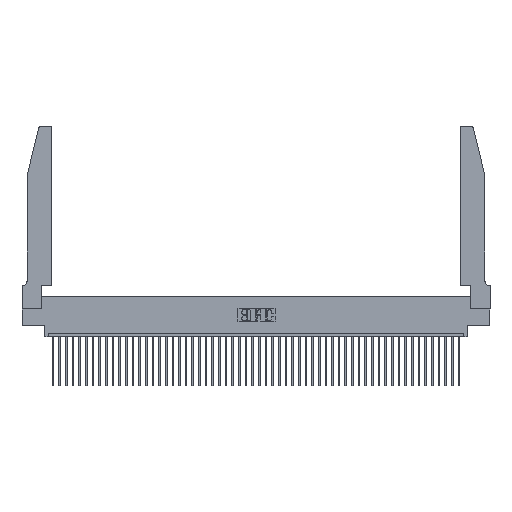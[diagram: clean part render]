
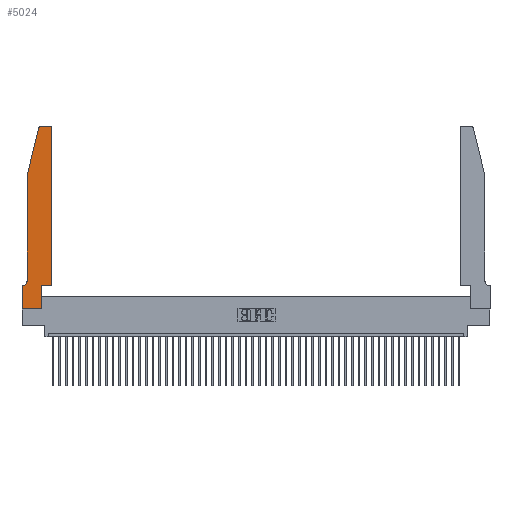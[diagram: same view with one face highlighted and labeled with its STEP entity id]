
A CAD part, top view. The second image highlights one B-rep face of the part: STEP entity #5024.
In plain terms, the highlighted planar face has unit normal (0, 0, 1).
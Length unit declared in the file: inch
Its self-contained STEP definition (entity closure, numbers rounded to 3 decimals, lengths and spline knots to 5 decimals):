
#981 = LINE ( 'NONE', #19259, #23423 ) ;
#1218 = CARTESIAN_POINT ( 'NONE',  ( 0.4205, 2.75, 0.37 ) ) ;
#2409 = LINE ( 'NONE', #38891, #30758 ) ;
#2956 = VERTEX_POINT ( 'NONE', #44778 ) ;
#4063 = LINE ( 'NONE', #10642, #10596 ) ;
#4858 = CARTESIAN_POINT ( 'NONE',  ( 0.0755, 0.42, 0.37 ) ) ;
#5024 = ADVANCED_FACE ( 'NONE', ( #37629 ), #31689, .T. ) ;
#5174 = AXIS2_PLACEMENT_3D ( 'NONE', #39821, #32008, #24219 ) ;
#5288 = CARTESIAN_POINT ( 'NONE',  ( 0.2605, 2.75, 0.37 ) ) ;
#5776 = ORIENTED_EDGE ( 'NONE', *, *, #29403, .T. ) ;
#6698 = CARTESIAN_POINT ( 'NONE',  ( 0.4505, 0.35, 0.37 ) ) ;
#6776 = EDGE_CURVE ( 'NONE', #11607, #11128, #981, .T. ) ;
#7155 = CARTESIAN_POINT ( 'NONE',  ( 0., 0., 0.37 ) ) ;
#7243 = EDGE_CURVE ( 'NONE', #45416, #43548, #16360, .T. ) ;
#7507 = VERTEX_POINT ( 'NONE', #24348 ) ;
#9375 = ORIENTED_EDGE ( 'NONE', *, *, #10533, .T. ) ;
#10142 = ORIENTED_EDGE ( 'NONE', *, *, #21286, .T. ) ;
#10409 = CARTESIAN_POINT ( 'NONE',  ( 0.25487, 2.72718, 0.37 ) ) ;
#10533 = EDGE_CURVE ( 'NONE', #43548, #13850, #2409, .T. ) ;
#10596 = VECTOR ( 'NONE', #25791, 39.37008 ) ;
#10642 = CARTESIAN_POINT ( 'NONE',  ( 0.2865, 0.35, 0.37 ) ) ;
#11128 = VERTEX_POINT ( 'NONE', #19359 ) ;
#11607 = VERTEX_POINT ( 'NONE', #10409 ) ;
#11941 = VECTOR ( 'NONE', #31706, 39.37008 ) ;
#12114 = ORIENTED_EDGE ( 'NONE', *, *, #33068, .T. ) ;
#12550 = LINE ( 'NONE', #29063, #44525 ) ;
#12596 = ORIENTED_EDGE ( 'NONE', *, *, #7243, .T. ) ;
#12612 = DIRECTION ( 'NONE',  ( 0., 0., 1. ) ) ;
#12664 = CIRCLE ( 'NONE', #46687, 0.03 ) ;
#13850 = VERTEX_POINT ( 'NONE', #18048 ) ;
#14382 = CARTESIAN_POINT ( 'NONE',  ( 0., 0.35, 0.37 ) ) ;
#15039 = ORIENTED_EDGE ( 'NONE', *, *, #22161, .T. ) ;
#15915 = DIRECTION ( 'NONE',  ( 1., 0., 0. ) ) ;
#16360 = LINE ( 'NONE', #6698, #35861 ) ;
#16865 = CARTESIAN_POINT ( 'NONE',  ( 0.2865, 0.35, 0.37 ) ) ;
#17271 = ORIENTED_EDGE ( 'NONE', *, *, #45090, .T. ) ;
#18048 = CARTESIAN_POINT ( 'NONE',  ( 0.4505, 2.72, 0.37 ) ) ;
#18105 = CARTESIAN_POINT ( 'NONE',  ( 0.4505, 0.35, 0.37 ) ) ;
#18521 = DIRECTION ( 'NONE',  ( 1., 0., 0. ) ) ;
#19259 = CARTESIAN_POINT ( 'NONE',  ( 0.0755, 2., 0.37 ) ) ;
#19359 = CARTESIAN_POINT ( 'NONE',  ( 0.0755, 2., 0.37 ) ) ;
#19743 = VERTEX_POINT ( 'NONE', #4858 ) ;
#20222 = VERTEX_POINT ( 'NONE', #1218 ) ;
#21286 = EDGE_CURVE ( 'NONE', #13850, #20222, #12664, .T. ) ;
#22161 = EDGE_CURVE ( 'NONE', #20222, #2956, #46835, .T. ) ;
#22281 = ORIENTED_EDGE ( 'NONE', *, *, #45531, .T. ) ;
#23395 = CIRCLE ( 'NONE', #42931, 0.03 ) ;
#23423 = VECTOR ( 'NONE', #41507, 39.37008 ) ;
#24219 = DIRECTION ( 'NONE',  ( 1., 0., 0. ) ) ;
#24348 = CARTESIAN_POINT ( 'NONE',  ( 0.2865, 0., 0.37 ) ) ;
#24536 = VECTOR ( 'NONE', #45156, 39.37008 ) ;
#24769 = CARTESIAN_POINT ( 'NONE',  ( 0.0755, 2., 0.37 ) ) ;
#25327 = LINE ( 'NONE', #7155, #41926 ) ;
#25791 = DIRECTION ( 'NONE',  ( 0., 1., 0. ) ) ;
#25943 = DIRECTION ( 'NONE',  ( 0., 0., 1. ) ) ;
#26003 = CARTESIAN_POINT ( 'NONE',  ( 0., 0., 0.37 ) ) ;
#27060 = CARTESIAN_POINT ( 'NONE',  ( 0.0055, 0.42, 0.37 ) ) ;
#27093 = ORIENTED_EDGE ( 'NONE', *, *, #32685, .T. ) ;
#27612 = CARTESIAN_POINT ( 'NONE',  ( 0.284, 2.72, 0.37 ) ) ;
#28756 = LINE ( 'NONE', #24769, #24536 ) ;
#29063 = CARTESIAN_POINT ( 'NONE',  ( 0.0755, 0.35, 0.37 ) ) ;
#29078 = DIRECTION ( 'NONE',  ( 1., 0., 0. ) ) ;
#29403 = EDGE_CURVE ( 'NONE', #19743, #30613, #37669, .T. ) ;
#30070 = ORIENTED_EDGE ( 'NONE', *, *, #6776, .T. ) ;
#30613 = VERTEX_POINT ( 'NONE', #31380 ) ;
#30758 = VECTOR ( 'NONE', #31578, 39.37008 ) ;
#30976 = VERTEX_POINT ( 'NONE', #26003 ) ;
#31380 = CARTESIAN_POINT ( 'NONE',  ( 0.0055, 0.35, 0.37 ) ) ;
#31578 = DIRECTION ( 'NONE',  ( 0., 1., 0. ) ) ;
#31689 = PLANE ( 'NONE',  #5174 ) ;
#31706 = DIRECTION ( 'NONE',  ( -1., 0., 0. ) ) ;
#31748 = ORIENTED_EDGE ( 'NONE', *, *, #41096, .T. ) ;
#32008 = DIRECTION ( 'NONE',  ( 0., 0., 1. ) ) ;
#32685 = EDGE_CURVE ( 'NONE', #34762, #30976, #34433, .T. ) ;
#33068 = EDGE_CURVE ( 'NONE', #30613, #34762, #12550, .T. ) ;
#34433 = LINE ( 'NONE', #42512, #41034 ) ;
#34528 = DIRECTION ( 'NONE',  ( 0., -1., 0. ) ) ;
#34762 = VERTEX_POINT ( 'NONE', #14382 ) ;
#34791 = AXIS2_PLACEMENT_3D ( 'NONE', #27060, #35001, #46088 ) ;
#35001 = DIRECTION ( 'NONE',  ( 0., 0., -1. ) ) ;
#35861 = VECTOR ( 'NONE', #36817, 39.37008 ) ;
#36398 = DIRECTION ( 'NONE',  ( -1., 0., 0. ) ) ;
#36817 = DIRECTION ( 'NONE',  ( 1., 0., 0. ) ) ;
#36916 = CARTESIAN_POINT ( 'NONE',  ( 0.4205, 2.72, 0.37 ) ) ;
#37629 = FACE_OUTER_BOUND ( 'NONE', #40304, .T. ) ;
#37669 = CIRCLE ( 'NONE', #34791, 0.07 ) ;
#38891 = CARTESIAN_POINT ( 'NONE',  ( 0.4505, 0.35, 0.37 ) ) ;
#39821 = CARTESIAN_POINT ( 'NONE',  ( 0., 0.35, 0.37 ) ) ;
#40304 = EDGE_LOOP ( 'NONE', ( #15039, #17271, #30070, #22281, #5776, #12114, #27093, #31748, #44744, #12596, #9375, #10142 ) ) ;
#41034 = VECTOR ( 'NONE', #34528, 39.37008 ) ;
#41068 = EDGE_CURVE ( 'NONE', #7507, #45416, #4063, .T. ) ;
#41096 = EDGE_CURVE ( 'NONE', #30976, #7507, #25327, .T. ) ;
#41507 = DIRECTION ( 'NONE',  ( -0.239, -0.971, 0. ) ) ;
#41926 = VECTOR ( 'NONE', #29078, 39.37008 ) ;
#42512 = CARTESIAN_POINT ( 'NONE',  ( 0., 0., 0.37 ) ) ;
#42931 = AXIS2_PLACEMENT_3D ( 'NONE', #27612, #12612, #15915 ) ;
#43548 = VERTEX_POINT ( 'NONE', #18105 ) ;
#44525 = VECTOR ( 'NONE', #36398, 39.37008 ) ;
#44744 = ORIENTED_EDGE ( 'NONE', *, *, #41068, .T. ) ;
#44778 = CARTESIAN_POINT ( 'NONE',  ( 0.284, 2.75, 0.37 ) ) ;
#45090 = EDGE_CURVE ( 'NONE', #2956, #11607, #23395, .T. ) ;
#45156 = DIRECTION ( 'NONE',  ( 0., -1., 0. ) ) ;
#45416 = VERTEX_POINT ( 'NONE', #16865 ) ;
#45531 = EDGE_CURVE ( 'NONE', #11128, #19743, #28756, .T. ) ;
#46088 = DIRECTION ( 'NONE',  ( -1., 0., 0. ) ) ;
#46687 = AXIS2_PLACEMENT_3D ( 'NONE', #36916, #25943, #18521 ) ;
#46835 = LINE ( 'NONE', #5288, #11941 ) ;
